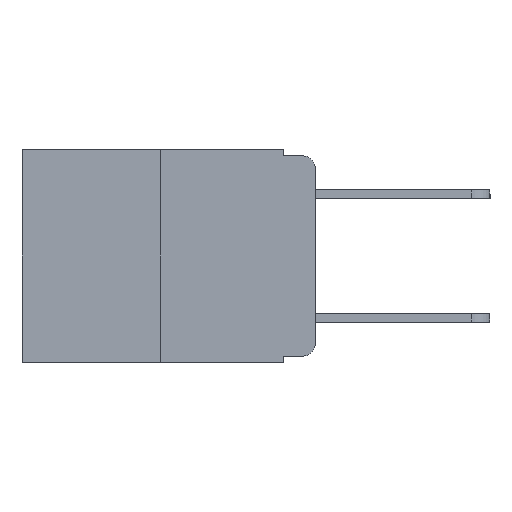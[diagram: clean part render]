
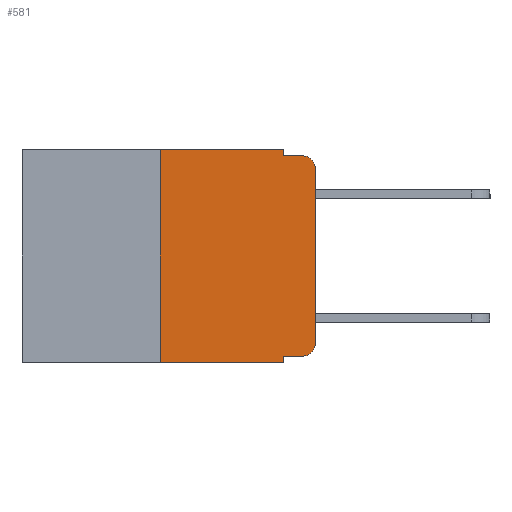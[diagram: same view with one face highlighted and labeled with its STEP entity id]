
A CAD part, left-side view. The second image highlights one B-rep face of the part: STEP entity #581.
In plain terms, the highlighted planar face has unit normal (-1, 0, 0).
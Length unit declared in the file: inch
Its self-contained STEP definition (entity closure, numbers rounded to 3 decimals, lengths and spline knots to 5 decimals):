
#138 = VERTEX_POINT ( 'NONE', #15509 ) ;
#429 = CARTESIAN_POINT ( 'NONE',  ( 0., 0.051, -0.333 ) ) ;
#581 = ADVANCED_FACE ( 'NONE', ( #12965 ), #4251, .F. ) ;
#1001 = VERTEX_POINT ( 'NONE', #11708 ) ;
#1273 = ORIENTED_EDGE ( 'NONE', *, *, #6671, .T. ) ;
#1422 = VECTOR ( 'NONE', #16436, 39.37008 ) ;
#1522 = VERTEX_POINT ( 'NONE', #9963 ) ;
#1719 = ORIENTED_EDGE ( 'NONE', *, *, #6413, .T. ) ;
#2410 = EDGE_LOOP ( 'NONE', ( #1273, #13894, #9675, #7462, #12775, #10520, #1719, #3076, #12605, #13011 ) ) ;
#2497 = CARTESIAN_POINT ( 'NONE',  ( 0., 0.051, -0.01 ) ) ;
#2642 = CARTESIAN_POINT ( 'NONE',  ( 0., 0.051, -0.333 ) ) ;
#2658 = EDGE_CURVE ( 'NONE', #11042, #1522, #4786, .T. ) ;
#2765 = DIRECTION ( 'NONE',  ( 0., -1., 0. ) ) ;
#2869 = LINE ( 'NONE', #5421, #9690 ) ;
#3076 = ORIENTED_EDGE ( 'NONE', *, *, #6728, .F. ) ;
#3309 = VECTOR ( 'NONE', #9342, 39.37008 ) ;
#4008 = CARTESIAN_POINT ( 'NONE',  ( 0., 0.25, 0. ) ) ;
#4124 = CARTESIAN_POINT ( 'NONE',  ( 0., 0.02, -0.313 ) ) ;
#4225 = CARTESIAN_POINT ( 'NONE',  ( 0., 0.473, 0. ) ) ;
#4251 = PLANE ( 'NONE',  #15772 ) ;
#4297 = VECTOR ( 'NONE', #2765, 39.37008 ) ;
#4378 = CARTESIAN_POINT ( 'NONE',  ( 0., 0.25, 0. ) ) ;
#4786 = LINE ( 'NONE', #4225, #4297 ) ;
#5330 = LINE ( 'NONE', #2642, #1422 ) ;
#5421 = CARTESIAN_POINT ( 'NONE',  ( 0., 0.051, 0. ) ) ;
#5615 = DIRECTION ( 'NONE',  ( 0., 0., -1. ) ) ;
#6187 = LINE ( 'NONE', #16643, #15433 ) ;
#6208 = LINE ( 'NONE', #4008, #9316 ) ;
#6413 = EDGE_CURVE ( 'NONE', #11004, #7224, #6187, .T. ) ;
#6590 = VERTEX_POINT ( 'NONE', #429 ) ;
#6641 = CIRCLE ( 'NONE', #9962, 0.02 ) ;
#6671 = EDGE_CURVE ( 'NONE', #1001, #16625, #13521, .T. ) ;
#6697 = EDGE_CURVE ( 'NONE', #16625, #138, #6641, .T. ) ;
#6700 = EDGE_CURVE ( 'NONE', #14578, #138, #10058, .T. ) ;
#6704 = EDGE_CURVE ( 'NONE', #1522, #14578, #2869, .T. ) ;
#6726 = EDGE_CURVE ( 'NONE', #11004, #11042, #6208, .T. ) ;
#6728 = EDGE_CURVE ( 'NONE', #6590, #7224, #16157, .T. ) ;
#6752 = EDGE_CURVE ( 'NONE', #6590, #8833, #5330, .T. ) ;
#6757 = EDGE_CURVE ( 'NONE', #8833, #1001, #15088, .T. ) ;
#6826 = DIRECTION ( 'NONE',  ( -1., 0., 0. ) ) ;
#6878 = DIRECTION ( 'NONE',  ( 0., 0., 1. ) ) ;
#7224 = VERTEX_POINT ( 'NONE', #13198 ) ;
#7462 = ORIENTED_EDGE ( 'NONE', *, *, #6704, .F. ) ;
#8048 = CARTESIAN_POINT ( 'NONE',  ( 0., 0., 0. ) ) ;
#8478 = DIRECTION ( 'NONE',  ( 0., -1., 0. ) ) ;
#8833 = VERTEX_POINT ( 'NONE', #14524 ) ;
#9316 = VECTOR ( 'NONE', #6878, 39.37008 ) ;
#9342 = DIRECTION ( 'NONE',  ( 0., 0., 1. ) ) ;
#9675 = ORIENTED_EDGE ( 'NONE', *, *, #6700, .F. ) ;
#9690 = VECTOR ( 'NONE', #16342, 39.37008 ) ;
#9707 = CARTESIAN_POINT ( 'NONE',  ( 0., 0.25, -0.343 ) ) ;
#9962 = AXIS2_PLACEMENT_3D ( 'NONE', #14046, #6826, #15184 ) ;
#9963 = CARTESIAN_POINT ( 'NONE',  ( 0., 0.051, 0. ) ) ;
#10058 = LINE ( 'NONE', #2497, #15814 ) ;
#10116 = CARTESIAN_POINT ( 'NONE',  ( 0., 0.051, -0.01 ) ) ;
#10520 = ORIENTED_EDGE ( 'NONE', *, *, #6726, .F. ) ;
#10573 = DIRECTION ( 'NONE',  ( 0., -1., 0. ) ) ;
#11004 = VERTEX_POINT ( 'NONE', #9707 ) ;
#11042 = VERTEX_POINT ( 'NONE', #4378 ) ;
#11708 = CARTESIAN_POINT ( 'NONE',  ( 0., 0., -0.313 ) ) ;
#12311 = AXIS2_PLACEMENT_3D ( 'NONE', #4124, #13081, #5615 ) ;
#12384 = DIRECTION ( 'NONE',  ( 1., 0., 0. ) ) ;
#12605 = ORIENTED_EDGE ( 'NONE', *, *, #6752, .T. ) ;
#12775 = ORIENTED_EDGE ( 'NONE', *, *, #2658, .F. ) ;
#12805 = VECTOR ( 'NONE', #16391, 39.37008 ) ;
#12965 = FACE_OUTER_BOUND ( 'NONE', #2410, .T. ) ;
#13011 = ORIENTED_EDGE ( 'NONE', *, *, #6757, .T. ) ;
#13081 = DIRECTION ( 'NONE',  ( -1., 0., 0. ) ) ;
#13198 = CARTESIAN_POINT ( 'NONE',  ( 0., 0.051, -0.343 ) ) ;
#13521 = LINE ( 'NONE', #8048, #3309 ) ;
#13591 = DIRECTION ( 'NONE',  ( 0., 0., -1. ) ) ;
#13894 = ORIENTED_EDGE ( 'NONE', *, *, #6697, .T. ) ;
#13957 = CARTESIAN_POINT ( 'NONE',  ( 0., 0., -0.03 ) ) ;
#14046 = CARTESIAN_POINT ( 'NONE',  ( 0., 0.02, -0.03 ) ) ;
#14524 = CARTESIAN_POINT ( 'NONE',  ( 0., 0.02, -0.333 ) ) ;
#14578 = VERTEX_POINT ( 'NONE', #10116 ) ;
#15088 = CIRCLE ( 'NONE', #12311, 0.02 ) ;
#15184 = DIRECTION ( 'NONE',  ( 0., 0., -1. ) ) ;
#15239 = CARTESIAN_POINT ( 'NONE',  ( 0., 0.051, 0. ) ) ;
#15433 = VECTOR ( 'NONE', #8478, 39.37008 ) ;
#15509 = CARTESIAN_POINT ( 'NONE',  ( 0., 0.02, -0.01 ) ) ;
#15772 = AXIS2_PLACEMENT_3D ( 'NONE', #16244, #12384, #13591 ) ;
#15814 = VECTOR ( 'NONE', #10573, 39.37008 ) ;
#16157 = LINE ( 'NONE', #15239, #12805 ) ;
#16244 = CARTESIAN_POINT ( 'NONE',  ( 0., 0.473, 0. ) ) ;
#16342 = DIRECTION ( 'NONE',  ( 0., 0., -1. ) ) ;
#16391 = DIRECTION ( 'NONE',  ( 0., 0., -1. ) ) ;
#16436 = DIRECTION ( 'NONE',  ( 0., -1., 0. ) ) ;
#16625 = VERTEX_POINT ( 'NONE', #13957 ) ;
#16643 = CARTESIAN_POINT ( 'NONE',  ( 0., 0.473, -0.343 ) ) ;
